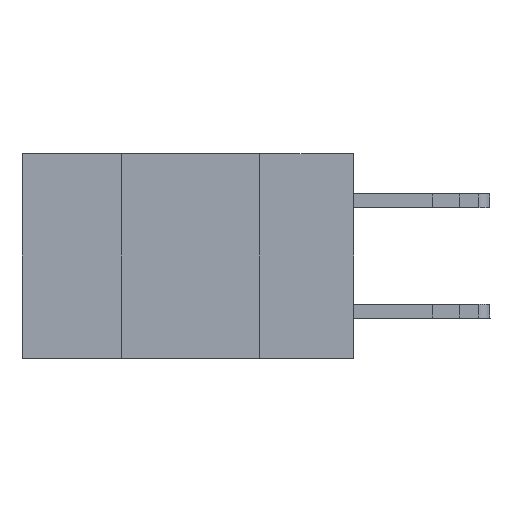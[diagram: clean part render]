
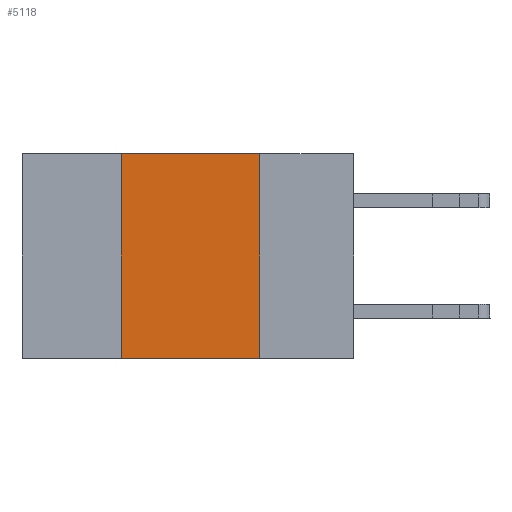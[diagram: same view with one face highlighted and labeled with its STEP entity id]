
A CAD part, left-side view. The second image highlights one B-rep face of the part: STEP entity #5118.
In plain terms, the highlighted planar face has unit normal (-1, 0, 0).
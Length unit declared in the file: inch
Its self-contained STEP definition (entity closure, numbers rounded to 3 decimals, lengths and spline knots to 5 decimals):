
#535 = DIRECTION ( 'NONE',  ( 0., -1., 0. ) ) ;
#1217 = ORIENTED_EDGE ( 'NONE', *, *, #9427, .F. ) ;
#1656 = PLANE ( 'NONE',  #20454 ) ;
#1744 = CARTESIAN_POINT ( 'NONE',  ( 0., 0.6, 0. ) ) ;
#3078 = VECTOR ( 'NONE', #535, 39.37008 ) ;
#3192 = EDGE_LOOP ( 'NONE', ( #13166, #1217, #3921, #9099 ) ) ;
#3921 = ORIENTED_EDGE ( 'NONE', *, *, #11522, .F. ) ;
#5066 = VECTOR ( 'NONE', #15451, 39.37008 ) ;
#5118 = ADVANCED_FACE ( 'NONE', ( #10014 ), #1656, .F. ) ;
#5176 = VECTOR ( 'NONE', #6522, 39.37008 ) ;
#5908 = VERTEX_POINT ( 'NONE', #12306 ) ;
#6002 = CARTESIAN_POINT ( 'NONE',  ( 0., 0.42, 0. ) ) ;
#6522 = DIRECTION ( 'NONE',  ( 0., -1., 0. ) ) ;
#7105 = DIRECTION ( 'NONE',  ( 1., 0., 0. ) ) ;
#7217 = CARTESIAN_POINT ( 'NONE',  ( 0., 0.42, 0. ) ) ;
#8246 = CARTESIAN_POINT ( 'NONE',  ( 0., 0.6, 0. ) ) ;
#8688 = VERTEX_POINT ( 'NONE', #6002 ) ;
#9099 = ORIENTED_EDGE ( 'NONE', *, *, #21074, .T. ) ;
#9234 = CARTESIAN_POINT ( 'NONE',  ( 0., 0.6, -0.37 ) ) ;
#9427 = EDGE_CURVE ( 'NONE', #8688, #19812, #15137, .T. ) ;
#10014 = FACE_OUTER_BOUND ( 'NONE', #3192, .T. ) ;
#10313 = CARTESIAN_POINT ( 'NONE',  ( 0., 0.17, 0. ) ) ;
#11522 = EDGE_CURVE ( 'NONE', #19084, #8688, #14021, .T. ) ;
#12248 = CARTESIAN_POINT ( 'NONE',  ( 0., 0.42, -0.37 ) ) ;
#12306 = CARTESIAN_POINT ( 'NONE',  ( 0., 0.17, -0.37 ) ) ;
#12649 = LINE ( 'NONE', #9234, #3078 ) ;
#13166 = ORIENTED_EDGE ( 'NONE', *, *, #15557, .F. ) ;
#14021 = LINE ( 'NONE', #7217, #5066 ) ;
#15137 = LINE ( 'NONE', #8246, #5176 ) ;
#15451 = DIRECTION ( 'NONE',  ( 0., 0., 1. ) ) ;
#15557 = EDGE_CURVE ( 'NONE', #19812, #5908, #19669, .T. ) ;
#15622 = CARTESIAN_POINT ( 'NONE',  ( 0., 0.17, 0. ) ) ;
#18129 = VECTOR ( 'NONE', #21831, 39.37008 ) ;
#18641 = DIRECTION ( 'NONE',  ( 0., 0., -1. ) ) ;
#19084 = VERTEX_POINT ( 'NONE', #12248 ) ;
#19669 = LINE ( 'NONE', #10313, #18129 ) ;
#19812 = VERTEX_POINT ( 'NONE', #15622 ) ;
#20454 = AXIS2_PLACEMENT_3D ( 'NONE', #1744, #7105, #18641 ) ;
#21074 = EDGE_CURVE ( 'NONE', #19084, #5908, #12649, .T. ) ;
#21831 = DIRECTION ( 'NONE',  ( 0., 0., -1. ) ) ;
